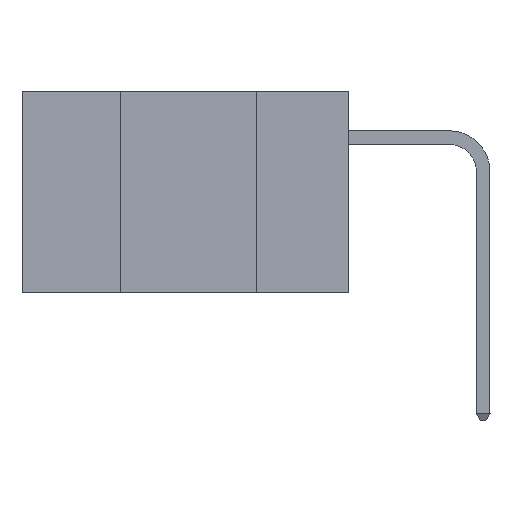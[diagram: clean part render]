
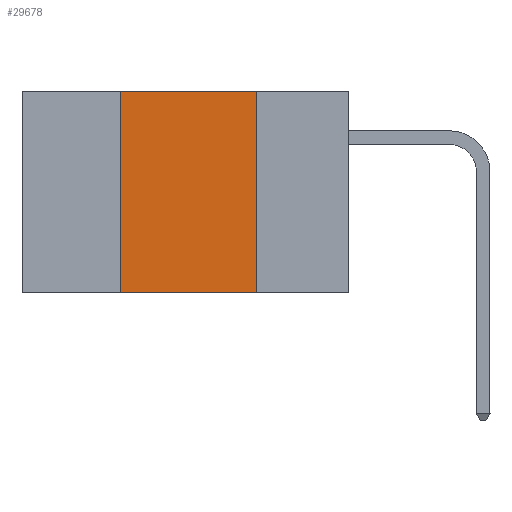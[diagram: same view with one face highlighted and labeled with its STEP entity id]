
A CAD part, left-side view. The second image highlights one B-rep face of the part: STEP entity #29678.
In plain terms, the highlighted planar face has unit normal (-1, 0, 0).
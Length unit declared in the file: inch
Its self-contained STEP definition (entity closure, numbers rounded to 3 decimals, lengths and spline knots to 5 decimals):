
#639 = CARTESIAN_POINT ( 'NONE',  ( 0., 0.17, 0. ) ) ;
#1602 = EDGE_CURVE ( 'NONE', #17515, #24107, #17345, .T. ) ;
#1892 = LINE ( 'NONE', #17040, #4615 ) ;
#2036 = DIRECTION ( 'NONE',  ( 0., 0., -1. ) ) ;
#2145 = ORIENTED_EDGE ( 'NONE', *, *, #1602, .F. ) ;
#2154 = ORIENTED_EDGE ( 'NONE', *, *, #12813, .F. ) ;
#3051 = FACE_OUTER_BOUND ( 'NONE', #17664, .T. ) ;
#3360 = CARTESIAN_POINT ( 'NONE',  ( 0., 0.6, 0. ) ) ;
#4021 = DIRECTION ( 'NONE',  ( 0., -1., 0. ) ) ;
#4615 = VECTOR ( 'NONE', #12215, 39.37008 ) ;
#7316 = VERTEX_POINT ( 'NONE', #19372 ) ;
#8574 = EDGE_CURVE ( 'NONE', #7316, #31228, #1892, .T. ) ;
#8811 = CARTESIAN_POINT ( 'NONE',  ( 0., 0.17, -0.37 ) ) ;
#11323 = VECTOR ( 'NONE', #2036, 39.37008 ) ;
#12009 = CARTESIAN_POINT ( 'NONE',  ( 0., 0.6, 0. ) ) ;
#12215 = DIRECTION ( 'NONE',  ( 0., -1., 0. ) ) ;
#12813 = EDGE_CURVE ( 'NONE', #7316, #17515, #31769, .T. ) ;
#13344 = DIRECTION ( 'NONE',  ( 1., 0., 0. ) ) ;
#14147 = DIRECTION ( 'NONE',  ( 0., 0., 1. ) ) ;
#15803 = LINE ( 'NONE', #639, #11323 ) ;
#17040 = CARTESIAN_POINT ( 'NONE',  ( 0., 0.6, -0.37 ) ) ;
#17345 = LINE ( 'NONE', #12009, #29046 ) ;
#17515 = VERTEX_POINT ( 'NONE', #24326 ) ;
#17664 = EDGE_LOOP ( 'NONE', ( #25189, #2145, #2154, #25624 ) ) ;
#19372 = CARTESIAN_POINT ( 'NONE',  ( 0., 0.42, -0.37 ) ) ;
#20677 = PLANE ( 'NONE',  #25371 ) ;
#21300 = DIRECTION ( 'NONE',  ( 0., 0., -1. ) ) ;
#21452 = VECTOR ( 'NONE', #14147, 39.37008 ) ;
#21775 = CARTESIAN_POINT ( 'NONE',  ( 0., 0.42, 0. ) ) ;
#24107 = VERTEX_POINT ( 'NONE', #31945 ) ;
#24152 = EDGE_CURVE ( 'NONE', #24107, #31228, #15803, .T. ) ;
#24326 = CARTESIAN_POINT ( 'NONE',  ( 0., 0.42, 0. ) ) ;
#25189 = ORIENTED_EDGE ( 'NONE', *, *, #24152, .F. ) ;
#25371 = AXIS2_PLACEMENT_3D ( 'NONE', #3360, #13344, #21300 ) ;
#25624 = ORIENTED_EDGE ( 'NONE', *, *, #8574, .T. ) ;
#29046 = VECTOR ( 'NONE', #4021, 39.37008 ) ;
#29678 = ADVANCED_FACE ( 'NONE', ( #3051 ), #20677, .F. ) ;
#31228 = VERTEX_POINT ( 'NONE', #8811 ) ;
#31769 = LINE ( 'NONE', #21775, #21452 ) ;
#31945 = CARTESIAN_POINT ( 'NONE',  ( 0., 0.17, 0. ) ) ;
